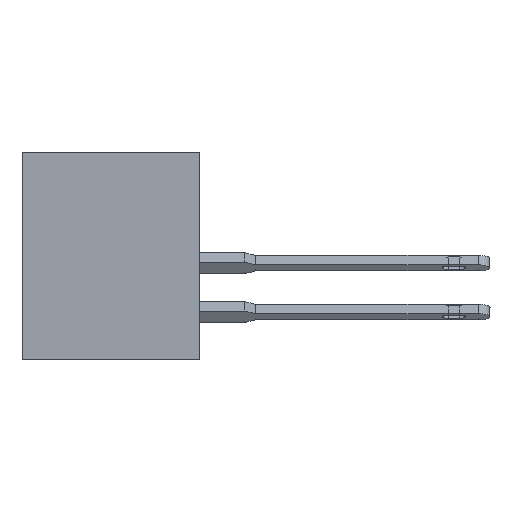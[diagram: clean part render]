
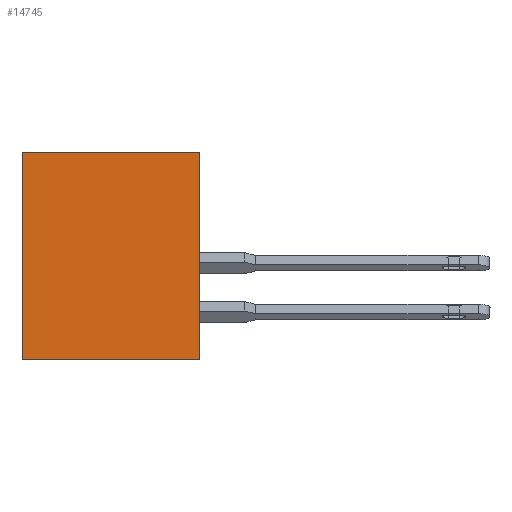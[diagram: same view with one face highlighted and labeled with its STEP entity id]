
A CAD part, left-side view. The second image highlights one B-rep face of the part: STEP entity #14745.
In plain terms, the highlighted planar face has unit normal (-1, 0, 0).
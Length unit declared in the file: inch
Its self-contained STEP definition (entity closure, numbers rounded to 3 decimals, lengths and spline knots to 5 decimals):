
#343 = CARTESIAN_POINT ( 'NONE',  ( 0., 0.453, 0. ) ) ;
#559 = EDGE_CURVE ( 'NONE', #5554, #11017, #8602, .T. ) ;
#580 = CARTESIAN_POINT ( 'NONE',  ( 0., 0.453, 0. ) ) ;
#785 = VECTOR ( 'NONE', #26608, 39.37008 ) ;
#1247 = VECTOR ( 'NONE', #8079, 39.37008 ) ;
#3562 = VECTOR ( 'NONE', #15032, 39.37008 ) ;
#4468 = EDGE_CURVE ( 'NONE', #11017, #19153, #19925, .T. ) ;
#4473 = DIRECTION ( 'NONE',  ( 0., 0., 1. ) ) ;
#5554 = VERTEX_POINT ( 'NONE', #9481 ) ;
#5889 = ORIENTED_EDGE ( 'NONE', *, *, #4468, .F. ) ;
#7031 = CARTESIAN_POINT ( 'NONE',  ( 0., 0.453, 0. ) ) ;
#8079 = DIRECTION ( 'NONE',  ( 0., 0., 1. ) ) ;
#8473 = DIRECTION ( 'NONE',  ( 0., 0., -1. ) ) ;
#8602 = LINE ( 'NONE', #343, #19565 ) ;
#9481 = CARTESIAN_POINT ( 'NONE',  ( 0., 0.453, -0.531 ) ) ;
#9954 = CARTESIAN_POINT ( 'NONE',  ( 0., 0., 0. ) ) ;
#11017 = VERTEX_POINT ( 'NONE', #7031 ) ;
#12813 = DIRECTION ( 'NONE',  ( 1., 0., 0. ) ) ;
#13556 = VERTEX_POINT ( 'NONE', #25484 ) ;
#14149 = CARTESIAN_POINT ( 'NONE',  ( 0., 0.453, -0.531 ) ) ;
#14745 = ADVANCED_FACE ( 'NONE', ( #16877 ), #24886, .F. ) ;
#15032 = DIRECTION ( 'NONE',  ( 0., -1., 0. ) ) ;
#15160 = EDGE_CURVE ( 'NONE', #5554, #13556, #15861, .T. ) ;
#15861 = LINE ( 'NONE', #14149, #785 ) ;
#16795 = ORIENTED_EDGE ( 'NONE', *, *, #559, .F. ) ;
#16877 = FACE_OUTER_BOUND ( 'NONE', #17880, .T. ) ;
#17880 = EDGE_LOOP ( 'NONE', ( #22062, #5889, #16795, #22551 ) ) ;
#19153 = VERTEX_POINT ( 'NONE', #24391 ) ;
#19565 = VECTOR ( 'NONE', #4473, 39.37008 ) ;
#19925 = LINE ( 'NONE', #580, #3562 ) ;
#20722 = CARTESIAN_POINT ( 'NONE',  ( 0., 0.453, 0. ) ) ;
#22062 = ORIENTED_EDGE ( 'NONE', *, *, #25798, .T. ) ;
#22551 = ORIENTED_EDGE ( 'NONE', *, *, #15160, .T. ) ;
#23130 = LINE ( 'NONE', #9954, #1247 ) ;
#24391 = CARTESIAN_POINT ( 'NONE',  ( 0., 0., 0. ) ) ;
#24886 = PLANE ( 'NONE',  #26168 ) ;
#25484 = CARTESIAN_POINT ( 'NONE',  ( 0., 0., -0.531 ) ) ;
#25798 = EDGE_CURVE ( 'NONE', #13556, #19153, #23130, .T. ) ;
#26168 = AXIS2_PLACEMENT_3D ( 'NONE', #20722, #12813, #8473 ) ;
#26608 = DIRECTION ( 'NONE',  ( 0., -1., 0. ) ) ;
